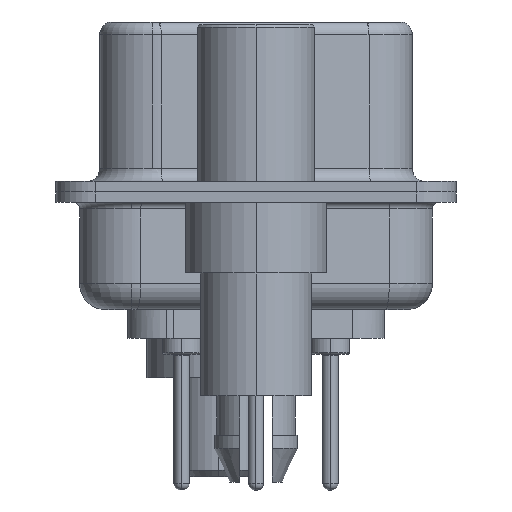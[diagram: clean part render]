
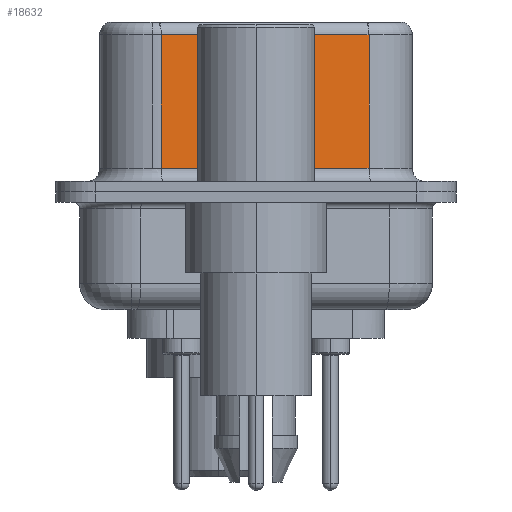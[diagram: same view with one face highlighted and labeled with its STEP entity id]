
A CAD part, left-side view. The second image highlights one B-rep face of the part: STEP entity #18632.
In plain terms, the highlighted planar face has unit normal (-0.985, -0.174, 0).
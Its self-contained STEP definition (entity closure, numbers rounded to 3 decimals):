
#1882 = LINE ( 'NONE', #17036, #28182 ) ;
#2370 = VERTEX_POINT ( 'NONE', #22833 ) ;
#2787 = CARTESIAN_POINT ( 'NONE',  ( 5.132, -4.322, 0.9 ) ) ;
#3722 = EDGE_CURVE ( 'NONE', #18241, #2370, #15262, .T. ) ;
#3948 = DIRECTION ( 'NONE',  ( 0., 0., -1. ) ) ;
#5001 = EDGE_CURVE ( 'NONE', #32345, #2370, #1882, .T. ) ;
#5364 = DIRECTION ( 'NONE',  ( 0.174, -0.985, 0. ) ) ;
#6305 = LINE ( 'NONE', #14320, #7119 ) ;
#6803 = EDGE_CURVE ( 'NONE', #32345, #31039, #22171, .T. ) ;
#6836 = ORIENTED_EDGE ( 'NONE', *, *, #15209, .T. ) ;
#7019 = ORIENTED_EDGE ( 'NONE', *, *, #3722, .T. ) ;
#7119 = VECTOR ( 'NONE', #3948, 1000. ) ;
#10549 = CARTESIAN_POINT ( 'NONE',  ( 3.73, 3.628, 0.9 ) ) ;
#10877 = CARTESIAN_POINT ( 'NONE',  ( 5.132, -4.322, 6.02 ) ) ;
#10938 = DIRECTION ( 'NONE',  ( -0.174, 0.985, 0. ) ) ;
#14320 = CARTESIAN_POINT ( 'NONE',  ( 3.73, 3.628, 6.52 ) ) ;
#14565 = DIRECTION ( 'NONE',  ( 0.985, 0.174, 0. ) ) ;
#15209 = EDGE_CURVE ( 'NONE', #31039, #18241, #6305, .T. ) ;
#15262 = LINE ( 'NONE', #2787, #27867 ) ;
#16240 = VECTOR ( 'NONE', #10938, 1000. ) ;
#17036 = CARTESIAN_POINT ( 'NONE',  ( 5.132, -4.322, 6.52 ) ) ;
#17785 = DIRECTION ( 'NONE',  ( 0., 0., -1. ) ) ;
#18241 = VERTEX_POINT ( 'NONE', #10549 ) ;
#18632 = ADVANCED_FACE ( 'NONE', ( #32753 ), #19535, .F. ) ;
#19535 = PLANE ( 'NONE',  #32681 ) ;
#20411 = ORIENTED_EDGE ( 'NONE', *, *, #6803, .T. ) ;
#22171 = LINE ( 'NONE', #10877, #16240 ) ;
#22510 = CARTESIAN_POINT ( 'NONE',  ( 5.132, -4.322, 6.02 ) ) ;
#22833 = CARTESIAN_POINT ( 'NONE',  ( 5.132, -4.322, 0.9 ) ) ;
#24554 = CARTESIAN_POINT ( 'NONE',  ( 3.73, 3.628, 6.02 ) ) ;
#27867 = VECTOR ( 'NONE', #5364, 1000. ) ;
#27874 = ORIENTED_EDGE ( 'NONE', *, *, #5001, .F. ) ;
#28182 = VECTOR ( 'NONE', #17785, 1000. ) ;
#29650 = CARTESIAN_POINT ( 'NONE',  ( 5.132, -4.322, 6.52 ) ) ;
#31039 = VERTEX_POINT ( 'NONE', #24554 ) ;
#31484 = EDGE_LOOP ( 'NONE', ( #27874, #20411, #6836, #7019 ) ) ;
#32241 = DIRECTION ( 'NONE',  ( -0.174, 0.985, 0. ) ) ;
#32345 = VERTEX_POINT ( 'NONE', #22510 ) ;
#32681 = AXIS2_PLACEMENT_3D ( 'NONE', #29650, #14565, #32241 ) ;
#32753 = FACE_OUTER_BOUND ( 'NONE', #31484, .T. ) ;
